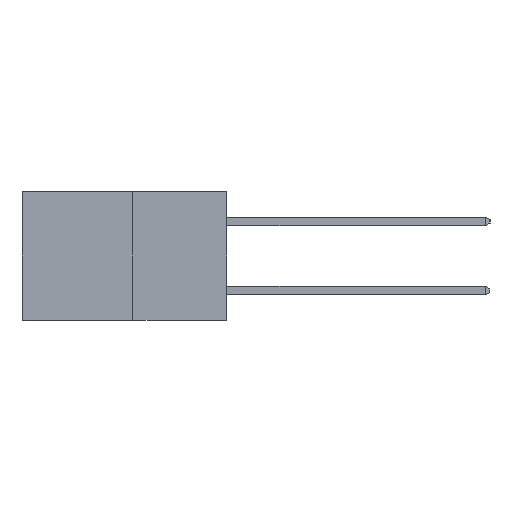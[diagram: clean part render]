
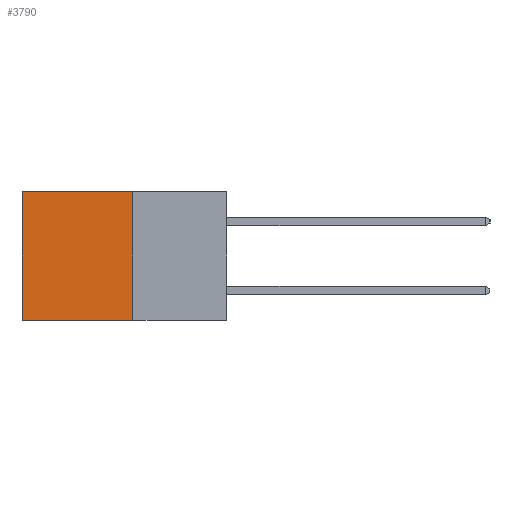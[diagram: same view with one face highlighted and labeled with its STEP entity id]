
A CAD part, left-side view. The second image highlights one B-rep face of the part: STEP entity #3790.
In plain terms, the highlighted planar face has unit normal (-1, 0, 0).
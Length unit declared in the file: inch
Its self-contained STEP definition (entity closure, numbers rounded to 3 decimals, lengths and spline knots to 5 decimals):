
#291 = FACE_OUTER_BOUND ( 'NONE', #1279, .T. ) ;
#351 = CARTESIAN_POINT ( 'NONE',  ( 0.277, 0.27, -0.37 ) ) ;
#1003 = EDGE_CURVE ( 'NONE', #5284, #7168, #3138, .T. ) ;
#1127 = DIRECTION ( 'NONE',  ( 0., 0., -1. ) ) ;
#1279 = EDGE_LOOP ( 'NONE', ( #8208, #3033, #3836, #4435 ) ) ;
#1492 = CARTESIAN_POINT ( 'NONE',  ( 0.277, 0.27, -0.37 ) ) ;
#1577 = VERTEX_POINT ( 'NONE', #351 ) ;
#2166 = DIRECTION ( 'NONE',  ( 0., 0., -1. ) ) ;
#2189 = CARTESIAN_POINT ( 'NONE',  ( 0.277, 0.59, -0.37 ) ) ;
#2788 = LINE ( 'NONE', #5804, #9273 ) ;
#3025 = CARTESIAN_POINT ( 'NONE',  ( 0.277, 0.27, 0. ) ) ;
#3033 = ORIENTED_EDGE ( 'NONE', *, *, #7862, .F. ) ;
#3138 = LINE ( 'NONE', #3753, #4615 ) ;
#3753 = CARTESIAN_POINT ( 'NONE',  ( 0.277, 0.27, 0. ) ) ;
#3790 = ADVANCED_FACE ( 'NONE', ( #291 ), #5190, .F. ) ;
#3836 = ORIENTED_EDGE ( 'NONE', *, *, #7962, .F. ) ;
#4032 = LINE ( 'NONE', #1492, #10361 ) ;
#4435 = ORIENTED_EDGE ( 'NONE', *, *, #1003, .T. ) ;
#4615 = VECTOR ( 'NONE', #10094, 39.37008 ) ;
#5035 = DIRECTION ( 'NONE',  ( 0., 0., -1. ) ) ;
#5146 = DIRECTION ( 'NONE',  ( 1., 0., 0. ) ) ;
#5171 = CARTESIAN_POINT ( 'NONE',  ( 0.277, 0.27, -0.37 ) ) ;
#5190 = PLANE ( 'NONE',  #7586 ) ;
#5284 = VERTEX_POINT ( 'NONE', #3025 ) ;
#5433 = EDGE_CURVE ( 'NONE', #7168, #8449, #8763, .T. ) ;
#5472 = DIRECTION ( 'NONE',  ( 0., 1., 0. ) ) ;
#5804 = CARTESIAN_POINT ( 'NONE',  ( 0.277, 0.27, -0.37 ) ) ;
#6514 = VECTOR ( 'NONE', #2166, 39.37008 ) ;
#6962 = CARTESIAN_POINT ( 'NONE',  ( 0.277, 0.59, 0. ) ) ;
#7072 = CARTESIAN_POINT ( 'NONE',  ( 0.277, 0.59, -0.37 ) ) ;
#7168 = VERTEX_POINT ( 'NONE', #6962 ) ;
#7586 = AXIS2_PLACEMENT_3D ( 'NONE', #5171, #5146, #5035 ) ;
#7862 = EDGE_CURVE ( 'NONE', #1577, #8449, #2788, .T. ) ;
#7962 = EDGE_CURVE ( 'NONE', #5284, #1577, #4032, .T. ) ;
#8208 = ORIENTED_EDGE ( 'NONE', *, *, #5433, .T. ) ;
#8449 = VERTEX_POINT ( 'NONE', #7072 ) ;
#8763 = LINE ( 'NONE', #2189, #6514 ) ;
#9273 = VECTOR ( 'NONE', #5472, 39.37008 ) ;
#10094 = DIRECTION ( 'NONE',  ( 0., 1., 0. ) ) ;
#10361 = VECTOR ( 'NONE', #1127, 39.37008 ) ;
